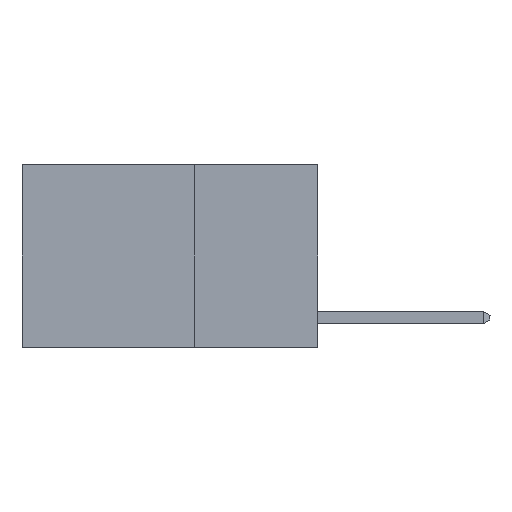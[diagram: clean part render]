
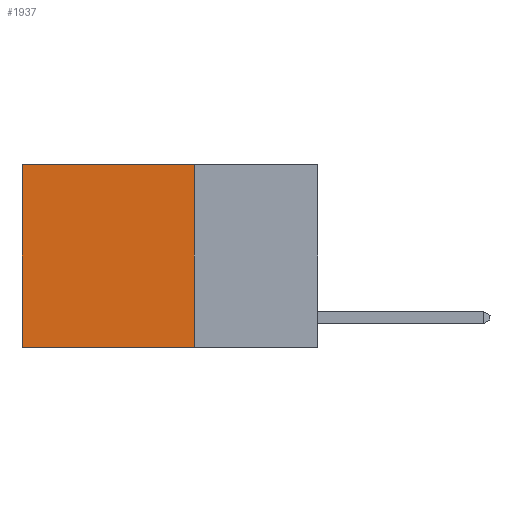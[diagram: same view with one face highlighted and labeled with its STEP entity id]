
A CAD part, left-side view. The second image highlights one B-rep face of the part: STEP entity #1937.
In plain terms, the highlighted planar face has unit normal (-1, 0, 0).
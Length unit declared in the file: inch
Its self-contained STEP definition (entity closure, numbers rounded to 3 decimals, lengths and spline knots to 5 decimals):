
#5 = FACE_OUTER_BOUND ( 'NONE', #8421, .T. ) ;
#10 = LINE ( 'NONE', #6881, #5033 ) ;
#201 = VERTEX_POINT ( 'NONE', #822 ) ;
#262 = ORIENTED_EDGE ( 'NONE', *, *, #2636, .T. ) ;
#822 = CARTESIAN_POINT ( 'NONE',  ( 0.2625, 0.25, 0. ) ) ;
#1076 = VECTOR ( 'NONE', #6961, 39.37008 ) ;
#1281 = CARTESIAN_POINT ( 'NONE',  ( 0.2625, 0.6, -0.37 ) ) ;
#1672 = ORIENTED_EDGE ( 'NONE', *, *, #1923, .F. ) ;
#1675 = VECTOR ( 'NONE', #4084, 39.37008 ) ;
#1923 = EDGE_CURVE ( 'NONE', #201, #2863, #3478, .T. ) ;
#1937 = ADVANCED_FACE ( 'NONE', ( #5 ), #4228, .F. ) ;
#1997 = DIRECTION ( 'NONE',  ( 0., 0., -1. ) ) ;
#2305 = DIRECTION ( 'NONE',  ( 0., 0., -1. ) ) ;
#2547 = CARTESIAN_POINT ( 'NONE',  ( 0.2625, 0.25, -0.37 ) ) ;
#2636 = EDGE_CURVE ( 'NONE', #8013, #6107, #8550, .T. ) ;
#2720 = CARTESIAN_POINT ( 'NONE',  ( 0.2625, 0.25, 0. ) ) ;
#2842 = CARTESIAN_POINT ( 'NONE',  ( 0.2625, 0.25, 0. ) ) ;
#2863 = VERTEX_POINT ( 'NONE', #2547 ) ;
#2961 = EDGE_CURVE ( 'NONE', #2863, #6107, #10, .T. ) ;
#3478 = LINE ( 'NONE', #2842, #1675 ) ;
#3860 = ORIENTED_EDGE ( 'NONE', *, *, #8183, .T. ) ;
#4084 = DIRECTION ( 'NONE',  ( 0., 0., -1. ) ) ;
#4134 = DIRECTION ( 'NONE',  ( 0., 1., 0. ) ) ;
#4171 = CARTESIAN_POINT ( 'NONE',  ( 0.2625, 0.25, 0. ) ) ;
#4181 = DIRECTION ( 'NONE',  ( 1., 0., 0. ) ) ;
#4228 = PLANE ( 'NONE',  #6655 ) ;
#4246 = ORIENTED_EDGE ( 'NONE', *, *, #2961, .F. ) ;
#5033 = VECTOR ( 'NONE', #4134, 39.37008 ) ;
#5499 = VECTOR ( 'NONE', #2305, 39.37008 ) ;
#5707 = CARTESIAN_POINT ( 'NONE',  ( 0.2625, 0.6, 0. ) ) ;
#5828 = CARTESIAN_POINT ( 'NONE',  ( 0.2625, 0.6, 0. ) ) ;
#6107 = VERTEX_POINT ( 'NONE', #1281 ) ;
#6224 = LINE ( 'NONE', #4171, #1076 ) ;
#6655 = AXIS2_PLACEMENT_3D ( 'NONE', #2720, #4181, #1997 ) ;
#6881 = CARTESIAN_POINT ( 'NONE',  ( 0.2625, 0.25, -0.37 ) ) ;
#6961 = DIRECTION ( 'NONE',  ( 0., 1., 0. ) ) ;
#8013 = VERTEX_POINT ( 'NONE', #5828 ) ;
#8183 = EDGE_CURVE ( 'NONE', #201, #8013, #6224, .T. ) ;
#8421 = EDGE_LOOP ( 'NONE', ( #262, #4246, #1672, #3860 ) ) ;
#8550 = LINE ( 'NONE', #5707, #5499 ) ;
